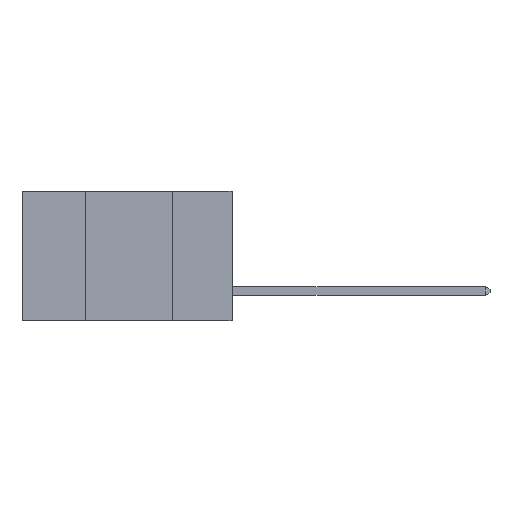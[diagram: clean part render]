
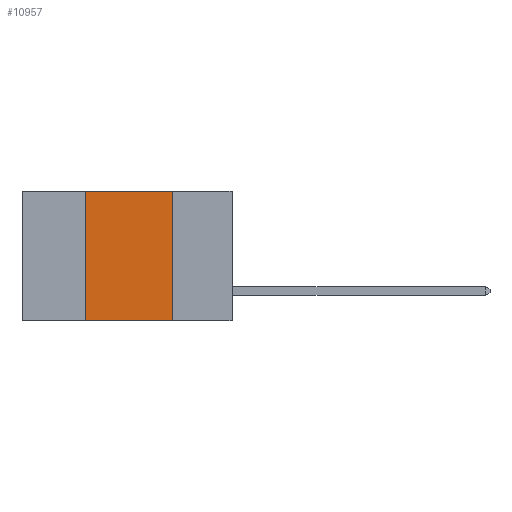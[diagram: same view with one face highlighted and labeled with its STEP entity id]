
A CAD part, left-side view. The second image highlights one B-rep face of the part: STEP entity #10957.
In plain terms, the highlighted planar face has unit normal (-1, 0, 0).
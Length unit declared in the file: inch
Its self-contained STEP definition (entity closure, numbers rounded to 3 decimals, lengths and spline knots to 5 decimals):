
#7 = DIRECTION ( 'NONE',  ( 0., -1., 0. ) ) ;
#963 = DIRECTION ( 'NONE',  ( 0., 0., 1. ) ) ;
#1435 = FACE_OUTER_BOUND ( 'NONE', #15388, .T. ) ;
#1903 = LINE ( 'NONE', #5343, #29195 ) ;
#2710 = VECTOR ( 'NONE', #13876, 39.37008 ) ;
#5093 = CARTESIAN_POINT ( 'NONE',  ( 0., 0.6, 0. ) ) ;
#5343 = CARTESIAN_POINT ( 'NONE',  ( 0., 0.6, 0. ) ) ;
#5788 = ORIENTED_EDGE ( 'NONE', *, *, #29092, .F. ) ;
#6404 = LINE ( 'NONE', #27747, #33540 ) ;
#10725 = VECTOR ( 'NONE', #963, 39.37008 ) ;
#10957 = ADVANCED_FACE ( 'NONE', ( #1435 ), #15887, .F. ) ;
#11128 = EDGE_CURVE ( 'NONE', #32954, #22848, #23911, .T. ) ;
#11290 = ORIENTED_EDGE ( 'NONE', *, *, #11128, .T. ) ;
#11691 = CARTESIAN_POINT ( 'NONE',  ( 0., 0.42, 0. ) ) ;
#12708 = EDGE_CURVE ( 'NONE', #33162, #22848, #6404, .T. ) ;
#13876 = DIRECTION ( 'NONE',  ( 0., -1., 0. ) ) ;
#15380 = EDGE_CURVE ( 'NONE', #32954, #21944, #17778, .T. ) ;
#15388 = EDGE_LOOP ( 'NONE', ( #24794, #5788, #19525, #11290 ) ) ;
#15551 = AXIS2_PLACEMENT_3D ( 'NONE', #5093, #34072, #18512 ) ;
#15887 = PLANE ( 'NONE',  #15551 ) ;
#17778 = LINE ( 'NONE', #11691, #10725 ) ;
#18512 = DIRECTION ( 'NONE',  ( 0., 0., -1. ) ) ;
#19525 = ORIENTED_EDGE ( 'NONE', *, *, #15380, .F. ) ;
#19965 = DIRECTION ( 'NONE',  ( 0., 0., -1. ) ) ;
#20924 = CARTESIAN_POINT ( 'NONE',  ( 0., 0.17, 0. ) ) ;
#21801 = CARTESIAN_POINT ( 'NONE',  ( 0., 0.17, -0.37 ) ) ;
#21944 = VERTEX_POINT ( 'NONE', #25410 ) ;
#22848 = VERTEX_POINT ( 'NONE', #21801 ) ;
#23911 = LINE ( 'NONE', #29538, #2710 ) ;
#24794 = ORIENTED_EDGE ( 'NONE', *, *, #12708, .F. ) ;
#25298 = CARTESIAN_POINT ( 'NONE',  ( 0., 0.42, -0.37 ) ) ;
#25410 = CARTESIAN_POINT ( 'NONE',  ( 0., 0.42, 0. ) ) ;
#27747 = CARTESIAN_POINT ( 'NONE',  ( 0., 0.17, 0. ) ) ;
#29092 = EDGE_CURVE ( 'NONE', #21944, #33162, #1903, .T. ) ;
#29195 = VECTOR ( 'NONE', #7, 39.37008 ) ;
#29538 = CARTESIAN_POINT ( 'NONE',  ( 0., 0.6, -0.37 ) ) ;
#32954 = VERTEX_POINT ( 'NONE', #25298 ) ;
#33162 = VERTEX_POINT ( 'NONE', #20924 ) ;
#33540 = VECTOR ( 'NONE', #19965, 39.37008 ) ;
#34072 = DIRECTION ( 'NONE',  ( 1., 0., 0. ) ) ;
